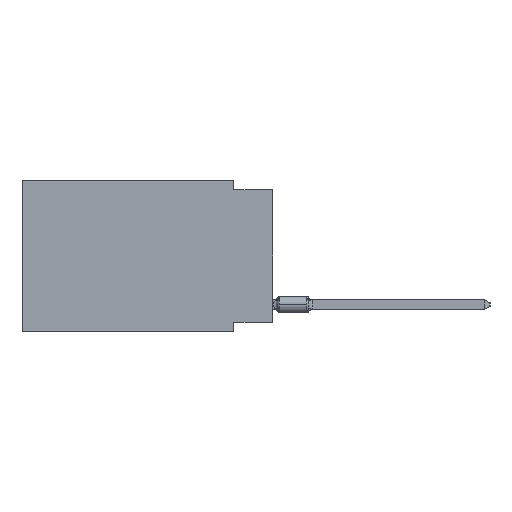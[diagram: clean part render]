
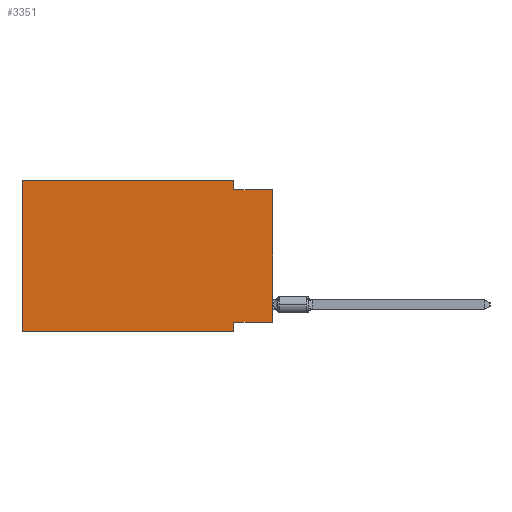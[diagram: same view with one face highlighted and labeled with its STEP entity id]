
A CAD part, left-side view. The second image highlights one B-rep face of the part: STEP entity #3351.
In plain terms, the highlighted planar face has unit normal (-1, 0, 0).
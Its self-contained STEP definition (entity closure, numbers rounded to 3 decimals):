
#80 = ORIENTED_EDGE ( 'NONE', *, *, #22333, .F. ) ;
#339 = ORIENTED_EDGE ( 'NONE', *, *, #15902, .F. ) ;
#648 = DIRECTION ( 'NONE',  ( 0., 0., 1. ) ) ;
#1317 = EDGE_CURVE ( 'NONE', #27626, #15519, #24597, .T. ) ;
#1923 = VERTEX_POINT ( 'NONE', #23079 ) ;
#2240 = LINE ( 'NONE', #12091, #5941 ) ;
#2536 = CARTESIAN_POINT ( 'NONE',  ( 0., 16.383, 0. ) ) ;
#3031 = VECTOR ( 'NONE', #648, 1000. ) ;
#3351 = ADVANCED_FACE ( 'NONE', ( #8020 ), #10272, .F. ) ;
#4813 = DIRECTION ( 'NONE',  ( 0., -1., 0. ) ) ;
#4971 = CARTESIAN_POINT ( 'NONE',  ( 0., 2.54, -9.906 ) ) ;
#5018 = VERTEX_POINT ( 'NONE', #23484 ) ;
#5200 = CARTESIAN_POINT ( 'NONE',  ( 0., 16.383, 0. ) ) ;
#5941 = VECTOR ( 'NONE', #4813, 1000. ) ;
#6314 = EDGE_CURVE ( 'NONE', #27626, #19348, #8076, .T. ) ;
#8020 = FACE_OUTER_BOUND ( 'NONE', #29872, .T. ) ;
#8076 = LINE ( 'NONE', #20693, #3031 ) ;
#8696 = CARTESIAN_POINT ( 'NONE',  ( 0., 0., -9.271 ) ) ;
#8941 = CARTESIAN_POINT ( 'NONE',  ( 0., 0., -0.635 ) ) ;
#9401 = CARTESIAN_POINT ( 'NONE',  ( 0., 16.383, -9.906 ) ) ;
#9470 = CARTESIAN_POINT ( 'NONE',  ( 0., 2.54, -9.906 ) ) ;
#9708 = DIRECTION ( 'NONE',  ( 0., -1., 0. ) ) ;
#9782 = CARTESIAN_POINT ( 'NONE',  ( 0., 16.383, -9.906 ) ) ;
#10272 = PLANE ( 'NONE',  #31956 ) ;
#10289 = VECTOR ( 'NONE', #28678, 1000. ) ;
#10331 = ORIENTED_EDGE ( 'NONE', *, *, #1317, .T. ) ;
#12091 = CARTESIAN_POINT ( 'NONE',  ( 0., 16.383, 0. ) ) ;
#12096 = LINE ( 'NONE', #4971, #17527 ) ;
#12644 = DIRECTION ( 'NONE',  ( 0., 0., 1. ) ) ;
#12708 = DIRECTION ( 'NONE',  ( 0., 0., -1. ) ) ;
#13508 = LINE ( 'NONE', #8941, #10289 ) ;
#15161 = EDGE_CURVE ( 'NONE', #5018, #15519, #12096, .T. ) ;
#15396 = CARTESIAN_POINT ( 'NONE',  ( 0., 0., 0. ) ) ;
#15519 = VERTEX_POINT ( 'NONE', #9470 ) ;
#15700 = DIRECTION ( 'NONE',  ( 0., 0., -1. ) ) ;
#15902 = EDGE_CURVE ( 'NONE', #1923, #18210, #13508, .T. ) ;
#15948 = DIRECTION ( 'NONE',  ( 0., 1., 0. ) ) ;
#16410 = ORIENTED_EDGE ( 'NONE', *, *, #28096, .F. ) ;
#17262 = DIRECTION ( 'NONE',  ( 0., 0., -1. ) ) ;
#17527 = VECTOR ( 'NONE', #17262, 1000. ) ;
#18210 = VERTEX_POINT ( 'NONE', #28881 ) ;
#19112 = VECTOR ( 'NONE', #12644, 1000. ) ;
#19348 = VERTEX_POINT ( 'NONE', #5200 ) ;
#19703 = CARTESIAN_POINT ( 'NONE',  ( 0., 2.54, 0. ) ) ;
#20693 = CARTESIAN_POINT ( 'NONE',  ( 0., 16.383, 0. ) ) ;
#21096 = ORIENTED_EDGE ( 'NONE', *, *, #30764, .T. ) ;
#21901 = ORIENTED_EDGE ( 'NONE', *, *, #6314, .F. ) ;
#22171 = VERTEX_POINT ( 'NONE', #8696 ) ;
#22333 = EDGE_CURVE ( 'NONE', #19348, #31466, #2240, .T. ) ;
#22889 = DIRECTION ( 'NONE',  ( 1., 0., 0. ) ) ;
#23079 = CARTESIAN_POINT ( 'NONE',  ( 0., 2.54, -0.635 ) ) ;
#23484 = CARTESIAN_POINT ( 'NONE',  ( 0., 2.54, -9.271 ) ) ;
#23722 = ORIENTED_EDGE ( 'NONE', *, *, #15161, .F. ) ;
#23948 = VECTOR ( 'NONE', #15948, 1000. ) ;
#24597 = LINE ( 'NONE', #9401, #25201 ) ;
#25201 = VECTOR ( 'NONE', #9708, 1000. ) ;
#26082 = EDGE_CURVE ( 'NONE', #31466, #1923, #30415, .T. ) ;
#27540 = ORIENTED_EDGE ( 'NONE', *, *, #26082, .F. ) ;
#27626 = VERTEX_POINT ( 'NONE', #9782 ) ;
#27849 = LINE ( 'NONE', #15396, #19112 ) ;
#27932 = CARTESIAN_POINT ( 'NONE',  ( 0., 0., -9.271 ) ) ;
#28096 = EDGE_CURVE ( 'NONE', #22171, #5018, #28235, .T. ) ;
#28235 = LINE ( 'NONE', #27932, #23948 ) ;
#28678 = DIRECTION ( 'NONE',  ( 0., -1., 0. ) ) ;
#28881 = CARTESIAN_POINT ( 'NONE',  ( 0., 0., -0.635 ) ) ;
#29872 = EDGE_LOOP ( 'NONE', ( #21096, #339, #27540, #80, #21901, #10331, #23722, #16410 ) ) ;
#30254 = CARTESIAN_POINT ( 'NONE',  ( 0., 2.54, 0. ) ) ;
#30415 = LINE ( 'NONE', #30254, #30798 ) ;
#30764 = EDGE_CURVE ( 'NONE', #22171, #18210, #27849, .T. ) ;
#30798 = VECTOR ( 'NONE', #15700, 1000. ) ;
#31466 = VERTEX_POINT ( 'NONE', #19703 ) ;
#31956 = AXIS2_PLACEMENT_3D ( 'NONE', #2536, #22889, #12708 ) ;
